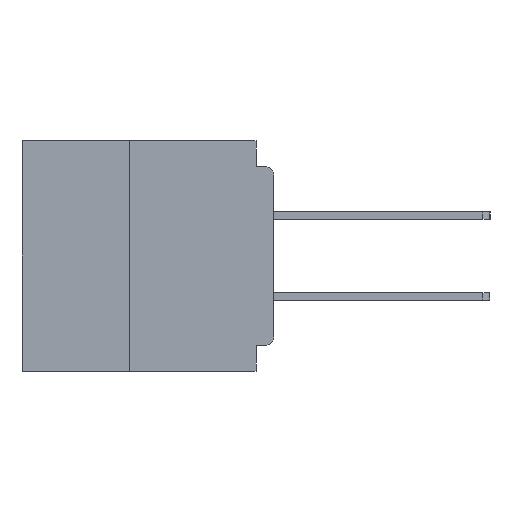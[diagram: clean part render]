
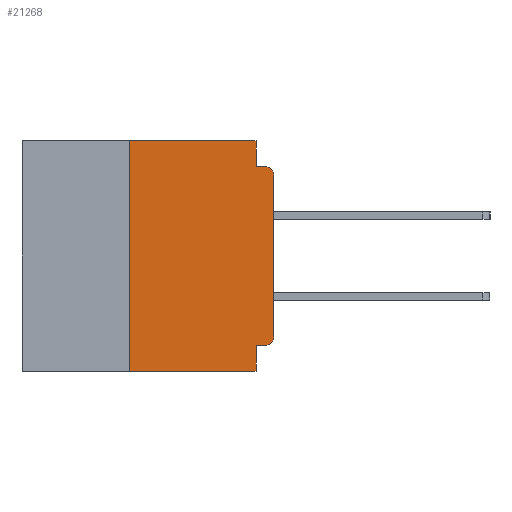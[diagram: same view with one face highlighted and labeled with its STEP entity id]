
A CAD part, left-side view. The second image highlights one B-rep face of the part: STEP entity #21268.
In plain terms, the highlighted planar face has unit normal (-1, 0, 0).
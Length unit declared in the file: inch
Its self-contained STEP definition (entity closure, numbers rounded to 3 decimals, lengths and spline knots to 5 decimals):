
#613 = CARTESIAN_POINT ( 'NONE',  ( 0., 0.031, 0. ) ) ;
#1250 = CARTESIAN_POINT ( 'NONE',  ( 0., 0., -0.06 ) ) ;
#2334 = EDGE_LOOP ( 'NONE', ( #20934, #41567, #12837, #41278, #38654, #6735, #34364, #16899, #27328, #37924 ) ) ;
#2524 = DIRECTION ( 'NONE',  ( 1., 0., 0. ) ) ;
#2707 = DIRECTION ( 'NONE',  ( 0., 1., 0. ) ) ;
#2780 = CARTESIAN_POINT ( 'NONE',  ( 0., 0.015, -0.355 ) ) ;
#2843 = VECTOR ( 'NONE', #47790, 39.37008 ) ;
#2989 = VERTEX_POINT ( 'NONE', #46222 ) ;
#3043 = DIRECTION ( 'NONE',  ( 0., -1., 0. ) ) ;
#3707 = EDGE_CURVE ( 'NONE', #31699, #40084, #4109, .T. ) ;
#4109 = LINE ( 'NONE', #38801, #33202 ) ;
#5271 = CARTESIAN_POINT ( 'NONE',  ( 0., 0.015, -0.34 ) ) ;
#5845 = CIRCLE ( 'NONE', #11682, 0.015 ) ;
#6341 = DIRECTION ( 'NONE',  ( 0., -1., 0. ) ) ;
#6501 = LINE ( 'NONE', #7856, #48413 ) ;
#6735 = ORIENTED_EDGE ( 'NONE', *, *, #41805, .F. ) ;
#7150 = FACE_OUTER_BOUND ( 'NONE', #2334, .T. ) ;
#7761 = VECTOR ( 'NONE', #6341, 39.37008 ) ;
#7856 = CARTESIAN_POINT ( 'NONE',  ( 0., 0.437, -0.4 ) ) ;
#8912 = DIRECTION ( 'NONE',  ( -1., 0., 0. ) ) ;
#9237 = DIRECTION ( 'NONE',  ( 0., 0., -1. ) ) ;
#9683 = DIRECTION ( 'NONE',  ( 0., 0., 1. ) ) ;
#10425 = CARTESIAN_POINT ( 'NONE',  ( 0., 0.437, 0. ) ) ;
#11682 = AXIS2_PLACEMENT_3D ( 'NONE', #5271, #32985, #9237 ) ;
#12837 = ORIENTED_EDGE ( 'NONE', *, *, #26897, .F. ) ;
#13668 = CARTESIAN_POINT ( 'NONE',  ( 0., 0.25, -0.4 ) ) ;
#14274 = EDGE_CURVE ( 'NONE', #25240, #45617, #28865, .T. ) ;
#14411 = PLANE ( 'NONE',  #50416 ) ;
#14922 = EDGE_CURVE ( 'NONE', #17469, #39835, #18891, .T. ) ;
#16899 = ORIENTED_EDGE ( 'NONE', *, *, #38052, .F. ) ;
#17469 = VERTEX_POINT ( 'NONE', #2780 ) ;
#17803 = EDGE_CURVE ( 'NONE', #40084, #2989, #38958, .T. ) ;
#17924 = VECTOR ( 'NONE', #3043, 39.37008 ) ;
#18110 = CARTESIAN_POINT ( 'NONE',  ( 0., 0.031, -0.045 ) ) ;
#18396 = DIRECTION ( 'NONE',  ( 0., 0., -1. ) ) ;
#18770 = CARTESIAN_POINT ( 'NONE',  ( 0., 0., -0.045 ) ) ;
#18891 = LINE ( 'NONE', #26363, #28173 ) ;
#19843 = DIRECTION ( 'NONE',  ( 0., -1., 0. ) ) ;
#20934 = ORIENTED_EDGE ( 'NONE', *, *, #3707, .T. ) ;
#21268 = ADVANCED_FACE ( 'NONE', ( #7150 ), #14411, .F. ) ;
#21570 = EDGE_CURVE ( 'NONE', #45617, #22431, #23833, .T. ) ;
#22081 = CARTESIAN_POINT ( 'NONE',  ( 0., 0., -0.34 ) ) ;
#22431 = VERTEX_POINT ( 'NONE', #18110 ) ;
#22494 = VECTOR ( 'NONE', #9683, 39.37008 ) ;
#23833 = LINE ( 'NONE', #613, #2843 ) ;
#25240 = VERTEX_POINT ( 'NONE', #38032 ) ;
#26363 = CARTESIAN_POINT ( 'NONE',  ( 0., 0., -0.355 ) ) ;
#26897 = EDGE_CURVE ( 'NONE', #22431, #2989, #28474, .T. ) ;
#27088 = DIRECTION ( 'NONE',  ( 0., 0., 1. ) ) ;
#27136 = VERTEX_POINT ( 'NONE', #43890 ) ;
#27328 = ORIENTED_EDGE ( 'NONE', *, *, #14922, .F. ) ;
#27875 = DIRECTION ( 'NONE',  ( 0., 0., -1. ) ) ;
#28044 = CARTESIAN_POINT ( 'NONE',  ( 0., 0.031, -0.4 ) ) ;
#28173 = VECTOR ( 'NONE', #2707, 39.37008 ) ;
#28474 = LINE ( 'NONE', #18770, #17924 ) ;
#28865 = LINE ( 'NONE', #45673, #7761 ) ;
#30409 = CARTESIAN_POINT ( 'NONE',  ( 0., 0.25, -0.4 ) ) ;
#31699 = VERTEX_POINT ( 'NONE', #22081 ) ;
#32650 = CARTESIAN_POINT ( 'NONE',  ( 0., 0.015, -0.06 ) ) ;
#32985 = DIRECTION ( 'NONE',  ( -1., 0., 0. ) ) ;
#33202 = VECTOR ( 'NONE', #27088, 39.37008 ) ;
#34364 = ORIENTED_EDGE ( 'NONE', *, *, #40902, .T. ) ;
#35871 = VECTOR ( 'NONE', #27875, 39.37008 ) ;
#36623 = DIRECTION ( 'NONE',  ( 0., 0., -1. ) ) ;
#37077 = LINE ( 'NONE', #28044, #35871 ) ;
#37924 = ORIENTED_EDGE ( 'NONE', *, *, #41133, .T. ) ;
#38032 = CARTESIAN_POINT ( 'NONE',  ( 0., 0.25, 0. ) ) ;
#38052 = EDGE_CURVE ( 'NONE', #39835, #27136, #37077, .T. ) ;
#38654 = ORIENTED_EDGE ( 'NONE', *, *, #14274, .F. ) ;
#38801 = CARTESIAN_POINT ( 'NONE',  ( 0., 0., 0. ) ) ;
#38958 = CIRCLE ( 'NONE', #44760, 0.015 ) ;
#39835 = VERTEX_POINT ( 'NONE', #46915 ) ;
#40084 = VERTEX_POINT ( 'NONE', #1250 ) ;
#40902 = EDGE_CURVE ( 'NONE', #46303, #27136, #6501, .T. ) ;
#41133 = EDGE_CURVE ( 'NONE', #17469, #31699, #5845, .T. ) ;
#41278 = ORIENTED_EDGE ( 'NONE', *, *, #21570, .F. ) ;
#41567 = ORIENTED_EDGE ( 'NONE', *, *, #17803, .T. ) ;
#41805 = EDGE_CURVE ( 'NONE', #46303, #25240, #43464, .T. ) ;
#43464 = LINE ( 'NONE', #13668, #22494 ) ;
#43890 = CARTESIAN_POINT ( 'NONE',  ( 0., 0.031, -0.4 ) ) ;
#44760 = AXIS2_PLACEMENT_3D ( 'NONE', #32650, #8912, #36623 ) ;
#45617 = VERTEX_POINT ( 'NONE', #50230 ) ;
#45673 = CARTESIAN_POINT ( 'NONE',  ( 0., 0.437, 0. ) ) ;
#46222 = CARTESIAN_POINT ( 'NONE',  ( 0., 0.015, -0.045 ) ) ;
#46303 = VERTEX_POINT ( 'NONE', #30409 ) ;
#46915 = CARTESIAN_POINT ( 'NONE',  ( 0., 0.031, -0.355 ) ) ;
#47790 = DIRECTION ( 'NONE',  ( 0., 0., -1. ) ) ;
#48413 = VECTOR ( 'NONE', #19843, 39.37008 ) ;
#50230 = CARTESIAN_POINT ( 'NONE',  ( 0., 0.031, 0. ) ) ;
#50416 = AXIS2_PLACEMENT_3D ( 'NONE', #10425, #2524, #18396 ) ;
